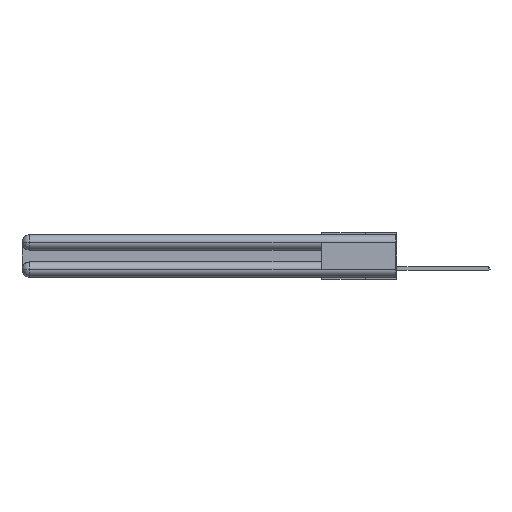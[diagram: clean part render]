
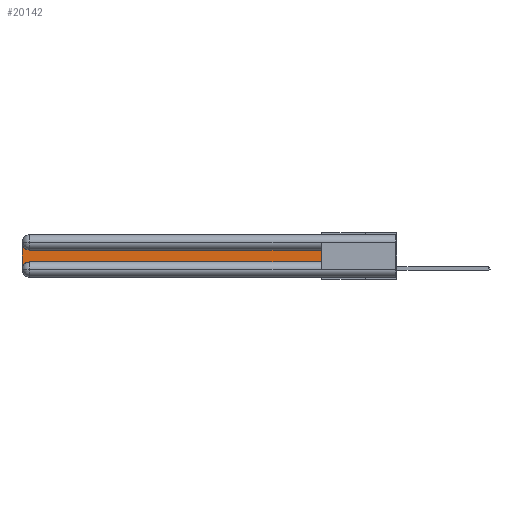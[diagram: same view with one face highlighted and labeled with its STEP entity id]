
A CAD part, left-side view. The second image highlights one B-rep face of the part: STEP entity #20142.
In plain terms, the highlighted planar face has unit normal (-1, 0, 0).
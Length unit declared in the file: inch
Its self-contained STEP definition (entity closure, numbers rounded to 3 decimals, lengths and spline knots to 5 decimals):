
#400 = CARTESIAN_POINT ( 'NONE',  ( 0.075, 0.6, -0.2175 ) ) ;
#672 = VECTOR ( 'NONE', #7012, 39.37008 ) ;
#1444 = EDGE_CURVE ( 'NONE', #16632, #28353, #14857, .T. ) ;
#2412 = VERTEX_POINT ( 'NONE', #18094 ) ;
#2814 = EDGE_CURVE ( 'NONE', #12881, #2412, #5657, .T. ) ;
#5078 = CARTESIAN_POINT ( 'NONE',  ( 0.075, 3., -0.2775 ) ) ;
#5127 = CARTESIAN_POINT ( 'NONE',  ( 0.075, 0.6, -0.2175 ) ) ;
#5285 = VECTOR ( 'NONE', #23757, 39.37008 ) ;
#5612 = ORIENTED_EDGE ( 'NONE', *, *, #19951, .T. ) ;
#5657 = LINE ( 'NONE', #22728, #5285 ) ;
#5841 = LINE ( 'NONE', #5127, #14933 ) ;
#6116 = AXIS2_PLACEMENT_3D ( 'NONE', #7671, #12519, #29488 ) ;
#7012 = DIRECTION ( 'NONE',  ( 0., 0., 1. ) ) ;
#7409 = CARTESIAN_POINT ( 'NONE',  ( 0.075, 3., -0.0625 ) ) ;
#7671 = CARTESIAN_POINT ( 'NONE',  ( 0.075, 3., -0.1225 ) ) ;
#7782 = CIRCLE ( 'NONE', #30276, 0.06 ) ;
#9683 = VECTOR ( 'NONE', #30803, 39.37008 ) ;
#10523 = ORIENTED_EDGE ( 'NONE', *, *, #1444, .T. ) ;
#10655 = ORIENTED_EDGE ( 'NONE', *, *, #27489, .T. ) ;
#11882 = DIRECTION ( 'NONE',  ( 1., 0., 0. ) ) ;
#12519 = DIRECTION ( 'NONE',  ( 1., 0., 0. ) ) ;
#12593 = AXIS2_PLACEMENT_3D ( 'NONE', #21228, #11882, #14209 ) ;
#12881 = VERTEX_POINT ( 'NONE', #21310 ) ;
#13680 = ORIENTED_EDGE ( 'NONE', *, *, #2814, .T. ) ;
#14209 = DIRECTION ( 'NONE',  ( 0., 0., -1. ) ) ;
#14610 = FACE_OUTER_BOUND ( 'NONE', #24224, .T. ) ;
#14649 = DIRECTION ( 'NONE',  ( 0., 0., -1. ) ) ;
#14744 = EDGE_CURVE ( 'NONE', #28353, #21873, #5841, .T. ) ;
#14857 = CIRCLE ( 'NONE', #12593, 0.06 ) ;
#14886 = DIRECTION ( 'NONE',  ( 0., -1., 0. ) ) ;
#14933 = VECTOR ( 'NONE', #14886, 39.37008 ) ;
#16632 = VERTEX_POINT ( 'NONE', #5078 ) ;
#16702 = CARTESIAN_POINT ( 'NONE',  ( 0.075, 3., -0.2175 ) ) ;
#18094 = CARTESIAN_POINT ( 'NONE',  ( 0.075, 2.94, -0.1225 ) ) ;
#19315 = DIRECTION ( 'NONE',  ( 1., 0., 0. ) ) ;
#19518 = EDGE_CURVE ( 'NONE', #22543, #16632, #22974, .T. ) ;
#19951 = EDGE_CURVE ( 'NONE', #2412, #22543, #7782, .T. ) ;
#20142 = ADVANCED_FACE ( 'NONE', ( #14610 ), #24713, .F. ) ;
#21228 = CARTESIAN_POINT ( 'NONE',  ( 0.075, 2.94, -0.2775 ) ) ;
#21310 = CARTESIAN_POINT ( 'NONE',  ( 0.075, 0.6, -0.1225 ) ) ;
#21478 = ORIENTED_EDGE ( 'NONE', *, *, #14744, .T. ) ;
#21873 = VERTEX_POINT ( 'NONE', #400 ) ;
#22271 = ORIENTED_EDGE ( 'NONE', *, *, #19518, .T. ) ;
#22543 = VERTEX_POINT ( 'NONE', #7409 ) ;
#22728 = CARTESIAN_POINT ( 'NONE',  ( 0.075, 0.6, -0.1225 ) ) ;
#22974 = LINE ( 'NONE', #16702, #9683 ) ;
#23757 = DIRECTION ( 'NONE',  ( 0., 1., 0. ) ) ;
#24224 = EDGE_LOOP ( 'NONE', ( #13680, #5612, #22271, #10523, #21478, #10655 ) ) ;
#24340 = CARTESIAN_POINT ( 'NONE',  ( 0.075, 2.94, -0.2175 ) ) ;
#24713 = PLANE ( 'NONE',  #6116 ) ;
#26498 = CARTESIAN_POINT ( 'NONE',  ( 0.075, 0.6, -0.2175 ) ) ;
#27489 = EDGE_CURVE ( 'NONE', #21873, #12881, #28393, .T. ) ;
#28353 = VERTEX_POINT ( 'NONE', #24340 ) ;
#28393 = LINE ( 'NONE', #26498, #672 ) ;
#29488 = DIRECTION ( 'NONE',  ( 0., 0., -1. ) ) ;
#30276 = AXIS2_PLACEMENT_3D ( 'NONE', #31308, #19315, #14649 ) ;
#30803 = DIRECTION ( 'NONE',  ( 0., 0., -1. ) ) ;
#31308 = CARTESIAN_POINT ( 'NONE',  ( 0.075, 2.94, -0.0625 ) ) ;
